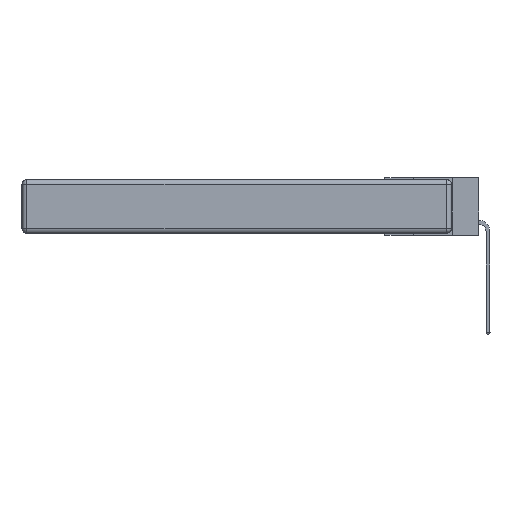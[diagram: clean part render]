
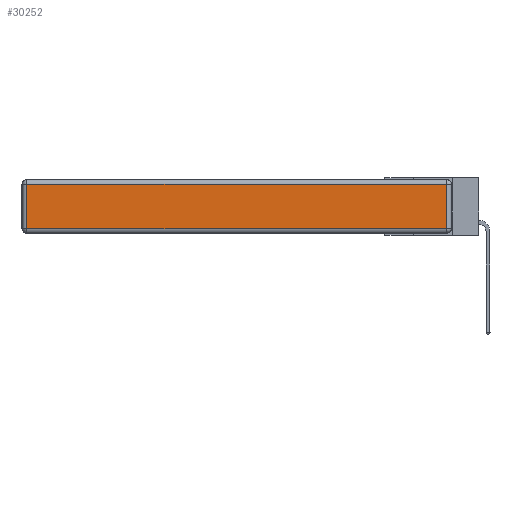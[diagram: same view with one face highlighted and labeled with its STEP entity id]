
A CAD part, left-side view. The second image highlights one B-rep face of the part: STEP entity #30252.
In plain terms, the highlighted planar face has unit normal (-1, 0, 0).
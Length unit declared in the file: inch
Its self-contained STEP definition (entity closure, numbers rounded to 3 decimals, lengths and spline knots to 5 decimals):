
#941 = EDGE_LOOP ( 'NONE', ( #16158, #19074, #10015, #20925 ) ) ;
#1480 = VECTOR ( 'NONE', #30082, 39.37008 ) ;
#1678 = VERTEX_POINT ( 'NONE', #30242 ) ;
#3722 = VERTEX_POINT ( 'NONE', #4779 ) ;
#4312 = DIRECTION ( 'NONE',  ( 0., 1., 0. ) ) ;
#4779 = CARTESIAN_POINT ( 'NONE',  ( 0., 0.03, -0.313 ) ) ;
#5791 = DIRECTION ( 'NONE',  ( 0., 0., 1. ) ) ;
#6577 = CARTESIAN_POINT ( 'NONE',  ( 0., 0., -0.313 ) ) ;
#8963 = EDGE_CURVE ( 'NONE', #1678, #15048, #17754, .T. ) ;
#9767 = VECTOR ( 'NONE', #5791, 39.37008 ) ;
#10015 = ORIENTED_EDGE ( 'NONE', *, *, #18785, .T. ) ;
#12437 = VECTOR ( 'NONE', #21442, 39.37008 ) ;
#13759 = EDGE_CURVE ( 'NONE', #15048, #3722, #31505, .T. ) ;
#15048 = VERTEX_POINT ( 'NONE', #18003 ) ;
#15352 = DIRECTION ( 'NONE',  ( 0., 0., 1. ) ) ;
#16158 = ORIENTED_EDGE ( 'NONE', *, *, #13759, .T. ) ;
#16370 = CARTESIAN_POINT ( 'NONE',  ( 0., 0.03, -0.343 ) ) ;
#17527 = EDGE_CURVE ( 'NONE', #3722, #23000, #28894, .T. ) ;
#17754 = LINE ( 'NONE', #26662, #12437 ) ;
#18003 = CARTESIAN_POINT ( 'NONE',  ( 0., 2.72, -0.313 ) ) ;
#18785 = EDGE_CURVE ( 'NONE', #23000, #1678, #28843, .T. ) ;
#19074 = ORIENTED_EDGE ( 'NONE', *, *, #17527, .T. ) ;
#20563 = FACE_OUTER_BOUND ( 'NONE', #941, .T. ) ;
#20925 = ORIENTED_EDGE ( 'NONE', *, *, #8963, .T. ) ;
#21146 = VECTOR ( 'NONE', #4312, 39.37008 ) ;
#21442 = DIRECTION ( 'NONE',  ( 0., 0., -1. ) ) ;
#23000 = VERTEX_POINT ( 'NONE', #24536 ) ;
#24536 = CARTESIAN_POINT ( 'NONE',  ( 0., 0.03, -0.03 ) ) ;
#25736 = PLANE ( 'NONE',  #27594 ) ;
#26662 = CARTESIAN_POINT ( 'NONE',  ( 0., 2.72, -0.343 ) ) ;
#27594 = AXIS2_PLACEMENT_3D ( 'NONE', #28339, #30900, #15352 ) ;
#28339 = CARTESIAN_POINT ( 'NONE',  ( 0., 0., -0.343 ) ) ;
#28843 = LINE ( 'NONE', #30420, #21146 ) ;
#28894 = LINE ( 'NONE', #16370, #9767 ) ;
#30082 = DIRECTION ( 'NONE',  ( 0., -1., 0. ) ) ;
#30242 = CARTESIAN_POINT ( 'NONE',  ( 0., 2.72, -0.03 ) ) ;
#30252 = ADVANCED_FACE ( 'NONE', ( #20563 ), #25736, .T. ) ;
#30420 = CARTESIAN_POINT ( 'NONE',  ( 0., 2.75, -0.03 ) ) ;
#30900 = DIRECTION ( 'NONE',  ( -1., 0., 0. ) ) ;
#31505 = LINE ( 'NONE', #6577, #1480 ) ;
